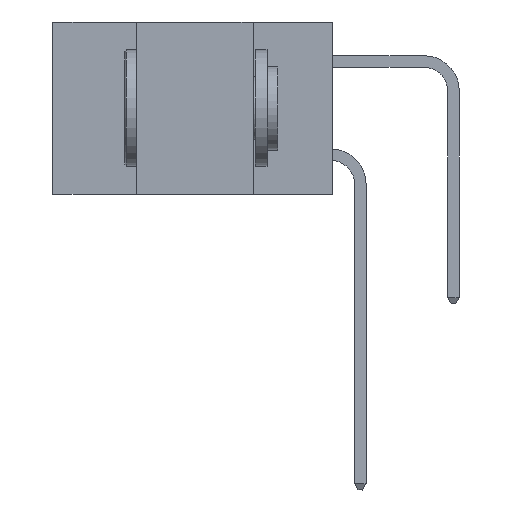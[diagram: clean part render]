
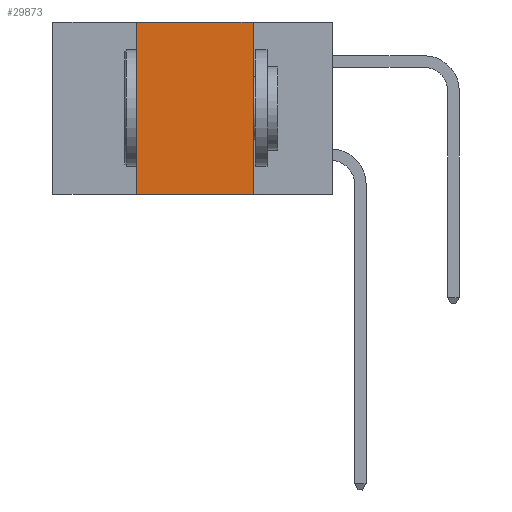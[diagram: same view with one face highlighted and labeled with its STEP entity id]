
A CAD part, left-side view. The second image highlights one B-rep face of the part: STEP entity #29873.
In plain terms, the highlighted planar face has unit normal (-1, 0, 0).
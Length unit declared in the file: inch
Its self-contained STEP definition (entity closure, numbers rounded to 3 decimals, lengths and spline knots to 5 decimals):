
#80 = ORIENTED_EDGE ( 'NONE', *, *, #11339, .T. ) ;
#3343 = AXIS2_PLACEMENT_3D ( 'NONE', #13253, #3829, #27718 ) ;
#3829 = DIRECTION ( 'NONE',  ( 1., 0., 0. ) ) ;
#4410 = DIRECTION ( 'NONE',  ( 0., -1., 0. ) ) ;
#5509 = VERTEX_POINT ( 'NONE', #26143 ) ;
#6642 = CARTESIAN_POINT ( 'NONE',  ( 0., 0.17, -0.37 ) ) ;
#6879 = FACE_OUTER_BOUND ( 'NONE', #22147, .T. ) ;
#8591 = ORIENTED_EDGE ( 'NONE', *, *, #8614, .F. ) ;
#8614 = EDGE_CURVE ( 'NONE', #5509, #25471, #18662, .T. ) ;
#8785 = DIRECTION ( 'NONE',  ( 0., 0., -1. ) ) ;
#8950 = LINE ( 'NONE', #15994, #25579 ) ;
#9777 = LINE ( 'NONE', #17327, #10531 ) ;
#10159 = VERTEX_POINT ( 'NONE', #28341 ) ;
#10531 = VECTOR ( 'NONE', #14302, 39.37008 ) ;
#11339 = EDGE_CURVE ( 'NONE', #18158, #25471, #19988, .T. ) ;
#11914 = CARTESIAN_POINT ( 'NONE',  ( 0., 0.6, -0.37 ) ) ;
#12086 = EDGE_CURVE ( 'NONE', #18158, #10159, #9777, .T. ) ;
#13253 = CARTESIAN_POINT ( 'NONE',  ( 0., 0.6, 0. ) ) ;
#14302 = DIRECTION ( 'NONE',  ( 0., 0., 1. ) ) ;
#15731 = CARTESIAN_POINT ( 'NONE',  ( 0., 0.17, 0. ) ) ;
#15862 = VECTOR ( 'NONE', #4410, 39.37008 ) ;
#15881 = PLANE ( 'NONE',  #3343 ) ;
#15994 = CARTESIAN_POINT ( 'NONE',  ( 0., 0.6, 0. ) ) ;
#17327 = CARTESIAN_POINT ( 'NONE',  ( 0., 0.42, 0. ) ) ;
#18158 = VERTEX_POINT ( 'NONE', #25756 ) ;
#18265 = VECTOR ( 'NONE', #8785, 39.37008 ) ;
#18662 = LINE ( 'NONE', #15731, #18265 ) ;
#19988 = LINE ( 'NONE', #11914, #15862 ) ;
#21174 = DIRECTION ( 'NONE',  ( 0., -1., 0. ) ) ;
#22147 = EDGE_LOOP ( 'NONE', ( #8591, #28812, #28046, #80 ) ) ;
#25471 = VERTEX_POINT ( 'NONE', #6642 ) ;
#25579 = VECTOR ( 'NONE', #21174, 39.37008 ) ;
#25756 = CARTESIAN_POINT ( 'NONE',  ( 0., 0.42, -0.37 ) ) ;
#26143 = CARTESIAN_POINT ( 'NONE',  ( 0., 0.17, 0. ) ) ;
#27134 = EDGE_CURVE ( 'NONE', #10159, #5509, #8950, .T. ) ;
#27718 = DIRECTION ( 'NONE',  ( 0., 0., -1. ) ) ;
#28046 = ORIENTED_EDGE ( 'NONE', *, *, #12086, .F. ) ;
#28341 = CARTESIAN_POINT ( 'NONE',  ( 0., 0.42, 0. ) ) ;
#28812 = ORIENTED_EDGE ( 'NONE', *, *, #27134, .F. ) ;
#29873 = ADVANCED_FACE ( 'NONE', ( #6879 ), #15881, .F. ) ;
